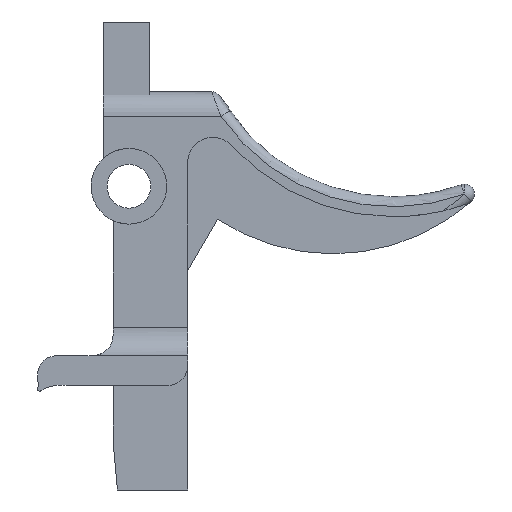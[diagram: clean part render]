
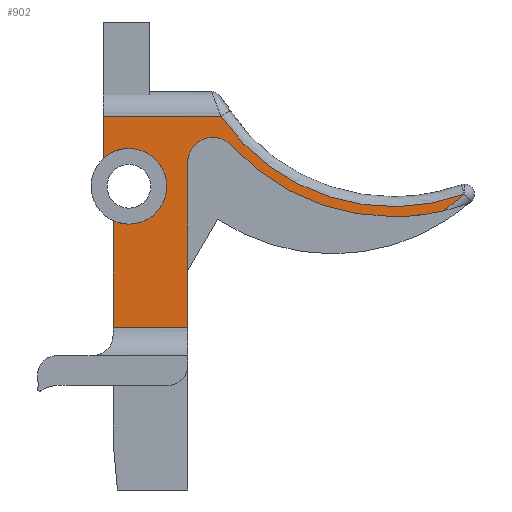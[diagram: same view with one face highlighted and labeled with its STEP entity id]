
A CAD part, left-side view. The second image highlights one B-rep face of the part: STEP entity #902.
In plain terms, the highlighted planar face has unit normal (-1, 0, 0).
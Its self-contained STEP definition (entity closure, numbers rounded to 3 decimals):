
#35 = VECTOR ( 'NONE', #1925, 1000. ) ;
#39 = EDGE_CURVE ( 'NONE', #437, #1082, #1580, .T. ) ;
#54 = VERTEX_POINT ( 'NONE', #248 ) ;
#68 = DIRECTION ( 'NONE',  ( -1., 0., 0. ) ) ;
#76 = LINE ( 'NONE', #982, #2188 ) ;
#100 = AXIS2_PLACEMENT_3D ( 'NONE', #603, #1425, #952 ) ;
#111 = ORIENTED_EDGE ( 'NONE', *, *, #112, .F. ) ;
#112 = EDGE_CURVE ( 'NONE', #1954, #1427, #1012, .T. ) ;
#136 = ORIENTED_EDGE ( 'NONE', *, *, #1031, .F. ) ;
#142 = EDGE_CURVE ( 'NONE', #2041, #54, #1970, .T. ) ;
#158 = CARTESIAN_POINT ( 'NONE',  ( -3.6, 0., -2.5 ) ) ;
#223 = EDGE_CURVE ( 'NONE', #2183, #973, #76, .T. ) ;
#248 = CARTESIAN_POINT ( 'NONE',  ( -3.6, -8.5, -7.135 ) ) ;
#268 = EDGE_CURVE ( 'NONE', #1082, #922, #1729, .T. ) ;
#314 = DIRECTION ( 'NONE',  ( 0., 0., 1. ) ) ;
#317 = CARTESIAN_POINT ( 'NONE',  ( -3.6, -8.5, -40. ) ) ;
#344 = VERTEX_POINT ( 'NONE', #2047 ) ;
#349 = PLANE ( 'NONE',  #1870 ) ;
#362 = ORIENTED_EDGE ( 'NONE', *, *, #39, .T. ) ;
#381 = CARTESIAN_POINT ( 'NONE',  ( -3.6, -36.296, -10.287 ) ) ;
#437 = VERTEX_POINT ( 'NONE', #1621 ) ;
#495 = DIRECTION ( 'NONE',  ( 0., 0., -1. ) ) ;
#517 = EDGE_CURVE ( 'NONE', #1427, #2139, #1098, .T. ) ;
#518 = DIRECTION ( 'NONE',  ( 1., 0., 0. ) ) ;
#571 = CARTESIAN_POINT ( 'NONE',  ( -3.6, -8.5, -23.672 ) ) ;
#596 = DIRECTION ( 'NONE',  ( 0., 0., 1. ) ) ;
#603 = CARTESIAN_POINT ( 'NONE',  ( -3.6, -29.126, 9.451 ) ) ;
#604 = AXIS2_PLACEMENT_3D ( 'NONE', #1943, #2122, #1611 ) ;
#688 = DIRECTION ( 'NONE',  ( 0., 0., 1. ) ) ;
#714 = ORIENTED_EDGE ( 'NONE', *, *, #1800, .T. ) ;
#715 = EDGE_CURVE ( 'NONE', #2139, #1665, #1837, .T. ) ;
#716 = CARTESIAN_POINT ( 'NONE',  ( -3.6, -23.074, -2.5 ) ) ;
#726 = CARTESIAN_POINT ( 'NONE',  ( -3.6, -11.858, -2.5 ) ) ;
#766 = CARTESIAN_POINT ( 'NONE',  ( -3.6, -1., -9.5 ) ) ;
#772 = VERTEX_POINT ( 'NONE', #158 ) ;
#798 = LINE ( 'NONE', #766, #1628 ) ;
#805 = ORIENTED_EDGE ( 'NONE', *, *, #1840, .F. ) ;
#809 = AXIS2_PLACEMENT_3D ( 'NONE', #2043, #518, #688 ) ;
#837 = DIRECTION ( 'NONE',  ( -1., 0., 0. ) ) ;
#872 = CARTESIAN_POINT ( 'NONE',  ( -3.6, -23.074, 4.719 ) ) ;
#883 = VECTOR ( 'NONE', #495, 1000. ) ;
#887 = CIRCLE ( 'NONE', #100, 22. ) ;
#901 = DIRECTION ( 'NONE',  ( 0., 0., 1. ) ) ;
#902 = ADVANCED_FACE ( 'NONE', ( #1045 ), #349, .T. ) ;
#922 = VERTEX_POINT ( 'NONE', #726 ) ;
#952 = DIRECTION ( 'NONE',  ( 0., 0., 1. ) ) ;
#973 = VERTEX_POINT ( 'NONE', #571 ) ;
#975 = DIRECTION ( 'NONE',  ( -1., 0., 0. ) ) ;
#982 = CARTESIAN_POINT ( 'NONE',  ( -3.6, -8.5, -23.672 ) ) ;
#1012 = CIRCLE ( 'NONE', #1418, 3.8 ) ;
#1031 = EDGE_CURVE ( 'NONE', #437, #344, #1652, .T. ) ;
#1035 = ORIENTED_EDGE ( 'NONE', *, *, #715, .F. ) ;
#1036 = CARTESIAN_POINT ( 'NONE',  ( -3.6, -1., -23.672 ) ) ;
#1045 = FACE_OUTER_BOUND ( 'NONE', #1247, .T. ) ;
#1057 = EDGE_CURVE ( 'NONE', #2183, #1954, #798, .T. ) ;
#1082 = VERTEX_POINT ( 'NONE', #381 ) ;
#1098 = CIRCLE ( 'NONE', #1664, 3.8 ) ;
#1113 = CARTESIAN_POINT ( 'NONE',  ( -3.6, -2.6, -9.5 ) ) ;
#1138 = CARTESIAN_POINT ( 'NONE',  ( -3.6, -2.6, -9.5 ) ) ;
#1174 = AXIS2_PLACEMENT_3D ( 'NONE', #1444, #1774, #1615 ) ;
#1226 = ORIENTED_EDGE ( 'NONE', *, *, #1057, .F. ) ;
#1247 = EDGE_LOOP ( 'NONE', ( #136, #362, #1278, #714, #1877, #1035, #1527, #111, #1226, #1821, #1863, #1426, #805 ) ) ;
#1249 = DIRECTION ( 'NONE',  ( -1., 0., 0. ) ) ;
#1278 = ORIENTED_EDGE ( 'NONE', *, *, #268, .T. ) ;
#1282 = DIRECTION ( 'NONE',  ( 0., 0., 1. ) ) ;
#1308 = DIRECTION ( 'NONE',  ( 0., 0., 1. ) ) ;
#1351 = DIRECTION ( 'NONE',  ( 0., 0., 1. ) ) ;
#1418 = AXIS2_PLACEMENT_3D ( 'NONE', #1113, #975, #1308 ) ;
#1425 = DIRECTION ( 'NONE',  ( 1., 0., 0. ) ) ;
#1426 = ORIENTED_EDGE ( 'NONE', *, *, #142, .F. ) ;
#1427 = VERTEX_POINT ( 'NONE', #2011 ) ;
#1443 = EDGE_CURVE ( 'NONE', #54, #973, #1607, .T. ) ;
#1444 = CARTESIAN_POINT ( 'NONE',  ( -3.6, -23.074, 4.719 ) ) ;
#1476 = DIRECTION ( 'NONE',  ( 0., 0., 1. ) ) ;
#1491 = CARTESIAN_POINT ( 'NONE',  ( -3.6, -12.912, -5.419 ) ) ;
#1493 = AXIS2_PLACEMENT_3D ( 'NONE', #2199, #837, #1351 ) ;
#1527 = ORIENTED_EDGE ( 'NONE', *, *, #517, .F. ) ;
#1536 = CARTESIAN_POINT ( 'NONE',  ( -3.6, -2.6, -5.7 ) ) ;
#1580 = CIRCLE ( 'NONE', #1174, 20. ) ;
#1601 = AXIS2_PLACEMENT_3D ( 'NONE', #1676, #2190, #1476 ) ;
#1607 = LINE ( 'NONE', #317, #883 ) ;
#1611 = DIRECTION ( 'NONE',  ( 0., 0., 1. ) ) ;
#1615 = DIRECTION ( 'NONE',  ( 0., 0., 1. ) ) ;
#1621 = CARTESIAN_POINT ( 'NONE',  ( -3.6, -34.072, -11.986 ) ) ;
#1623 = CARTESIAN_POINT ( 'NONE',  ( -3.6, -1., -12.947 ) ) ;
#1628 = VECTOR ( 'NONE', #314, 1000. ) ;
#1652 = CIRCLE ( 'NONE', #604, 22. ) ;
#1655 = LINE ( 'NONE', #1743, #1841 ) ;
#1664 = AXIS2_PLACEMENT_3D ( 'NONE', #1138, #68, #1282 ) ;
#1665 = VERTEX_POINT ( 'NONE', #1901 ) ;
#1676 = CARTESIAN_POINT ( 'NONE',  ( -3.6, -11.04, -7.135 ) ) ;
#1729 = CIRCLE ( 'NONE', #809, 21. ) ;
#1743 = CARTESIAN_POINT ( 'NONE',  ( -3.6, 0., 0. ) ) ;
#1753 = EDGE_CURVE ( 'NONE', #1665, #772, #1655, .T. ) ;
#1774 = DIRECTION ( 'NONE',  ( -1., 0., 0. ) ) ;
#1800 = EDGE_CURVE ( 'NONE', #922, #772, #1903, .T. ) ;
#1821 = ORIENTED_EDGE ( 'NONE', *, *, #223, .T. ) ;
#1837 = CIRCLE ( 'NONE', #1493, 3.8 ) ;
#1840 = EDGE_CURVE ( 'NONE', #344, #2041, #887, .T. ) ;
#1841 = VECTOR ( 'NONE', #901, 1000. ) ;
#1863 = ORIENTED_EDGE ( 'NONE', *, *, #1443, .F. ) ;
#1870 = AXIS2_PLACEMENT_3D ( 'NONE', #872, #1249, #596 ) ;
#1877 = ORIENTED_EDGE ( 'NONE', *, *, #1753, .F. ) ;
#1901 = CARTESIAN_POINT ( 'NONE',  ( -3.6, 0., -6.729 ) ) ;
#1903 = LINE ( 'NONE', #716, #35 ) ;
#1925 = DIRECTION ( 'NONE',  ( 0., 1., 0. ) ) ;
#1943 = CARTESIAN_POINT ( 'NONE',  ( -3.6, -29.126, 9.451 ) ) ;
#1954 = VERTEX_POINT ( 'NONE', #1623 ) ;
#1970 = CIRCLE ( 'NONE', #1601, 2.54 ) ;
#2011 = CARTESIAN_POINT ( 'NONE',  ( -3.6, -2.6, -13.3 ) ) ;
#2026 = DIRECTION ( 'NONE',  ( 0., -1., 0. ) ) ;
#2041 = VERTEX_POINT ( 'NONE', #1491 ) ;
#2043 = CARTESIAN_POINT ( 'NONE',  ( -3.6, -29.126, 9.451 ) ) ;
#2047 = CARTESIAN_POINT ( 'NONE',  ( -3.6, -29.126, -12.549 ) ) ;
#2122 = DIRECTION ( 'NONE',  ( 1., 0., 0. ) ) ;
#2139 = VERTEX_POINT ( 'NONE', #1536 ) ;
#2183 = VERTEX_POINT ( 'NONE', #1036 ) ;
#2188 = VECTOR ( 'NONE', #2026, 1000. ) ;
#2190 = DIRECTION ( 'NONE',  ( -1., 0., 0. ) ) ;
#2199 = CARTESIAN_POINT ( 'NONE',  ( -3.6, -2.6, -9.5 ) ) ;
